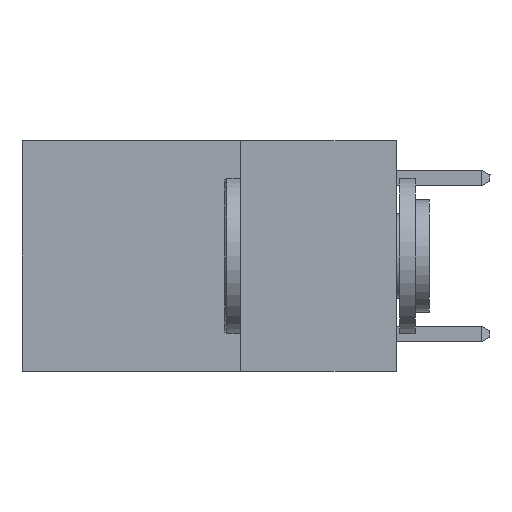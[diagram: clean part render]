
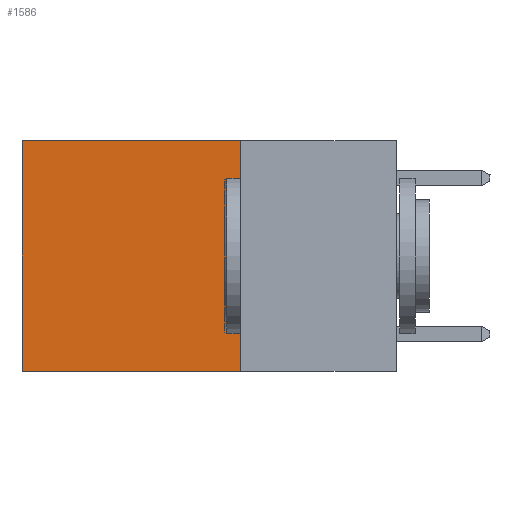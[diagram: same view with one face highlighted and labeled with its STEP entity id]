
A CAD part, left-side view. The second image highlights one B-rep face of the part: STEP entity #1586.
In plain terms, the highlighted planar face has unit normal (-1, 0, 0).
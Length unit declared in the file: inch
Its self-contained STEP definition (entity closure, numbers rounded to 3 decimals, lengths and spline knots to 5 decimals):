
#451 = VECTOR ( 'NONE', #22688, 39.37008 ) ;
#785 = CARTESIAN_POINT ( 'NONE',  ( 0.2625, 0.25, 0. ) ) ;
#1359 = CARTESIAN_POINT ( 'NONE',  ( 0.2625, 0.25, 0. ) ) ;
#1586 = ADVANCED_FACE ( 'NONE', ( #4761 ), #5731, .F. ) ;
#2191 = VERTEX_POINT ( 'NONE', #5698 ) ;
#3033 = ORIENTED_EDGE ( 'NONE', *, *, #21089, .F. ) ;
#3394 = EDGE_CURVE ( 'NONE', #4273, #2191, #7879, .T. ) ;
#4273 = VERTEX_POINT ( 'NONE', #19488 ) ;
#4579 = EDGE_LOOP ( 'NONE', ( #14478, #3033, #20928, #7301 ) ) ;
#4761 = FACE_OUTER_BOUND ( 'NONE', #4579, .T. ) ;
#5698 = CARTESIAN_POINT ( 'NONE',  ( 0.2625, 0.6, -0.37 ) ) ;
#5731 = PLANE ( 'NONE',  #7546 ) ;
#5841 = LINE ( 'NONE', #1359, #451 ) ;
#7301 = ORIENTED_EDGE ( 'NONE', *, *, #17246, .T. ) ;
#7546 = AXIS2_PLACEMENT_3D ( 'NONE', #11458, #19143, #7673 ) ;
#7601 = VECTOR ( 'NONE', #22685, 39.37008 ) ;
#7673 = DIRECTION ( 'NONE',  ( 0., 0., -1. ) ) ;
#7879 = LINE ( 'NONE', #20779, #7601 ) ;
#8317 = VECTOR ( 'NONE', #16689, 39.37008 ) ;
#8568 = DIRECTION ( 'NONE',  ( 0., 1., 0. ) ) ;
#10417 = CARTESIAN_POINT ( 'NONE',  ( 0.2625, 0.25, -0.37 ) ) ;
#11458 = CARTESIAN_POINT ( 'NONE',  ( 0.2625, 0.25, 0. ) ) ;
#12358 = EDGE_CURVE ( 'NONE', #19126, #16541, #5841, .T. ) ;
#14478 = ORIENTED_EDGE ( 'NONE', *, *, #3394, .T. ) ;
#14762 = CARTESIAN_POINT ( 'NONE',  ( 0.2625, 0.25, 0. ) ) ;
#16541 = VERTEX_POINT ( 'NONE', #22263 ) ;
#16689 = DIRECTION ( 'NONE',  ( 0., 1., 0. ) ) ;
#17246 = EDGE_CURVE ( 'NONE', #19126, #4273, #23249, .T. ) ;
#19126 = VERTEX_POINT ( 'NONE', #785 ) ;
#19143 = DIRECTION ( 'NONE',  ( 1., 0., 0. ) ) ;
#19488 = CARTESIAN_POINT ( 'NONE',  ( 0.2625, 0.6, 0. ) ) ;
#20779 = CARTESIAN_POINT ( 'NONE',  ( 0.2625, 0.6, 0. ) ) ;
#20928 = ORIENTED_EDGE ( 'NONE', *, *, #12358, .F. ) ;
#21089 = EDGE_CURVE ( 'NONE', #16541, #2191, #22036, .T. ) ;
#21435 = VECTOR ( 'NONE', #8568, 39.37008 ) ;
#22036 = LINE ( 'NONE', #10417, #21435 ) ;
#22263 = CARTESIAN_POINT ( 'NONE',  ( 0.2625, 0.25, -0.37 ) ) ;
#22685 = DIRECTION ( 'NONE',  ( 0., 0., -1. ) ) ;
#22688 = DIRECTION ( 'NONE',  ( 0., 0., -1. ) ) ;
#23249 = LINE ( 'NONE', #14762, #8317 ) ;
